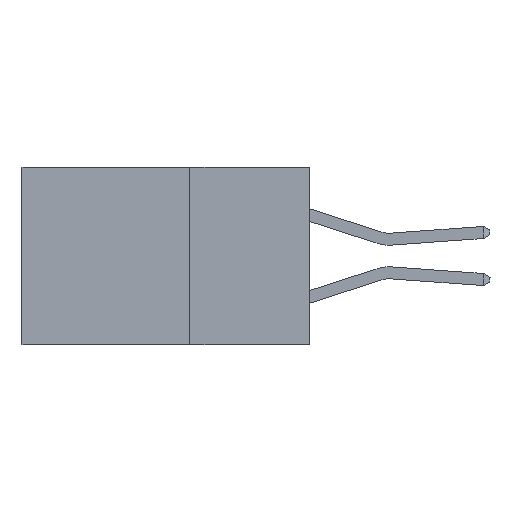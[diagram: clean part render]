
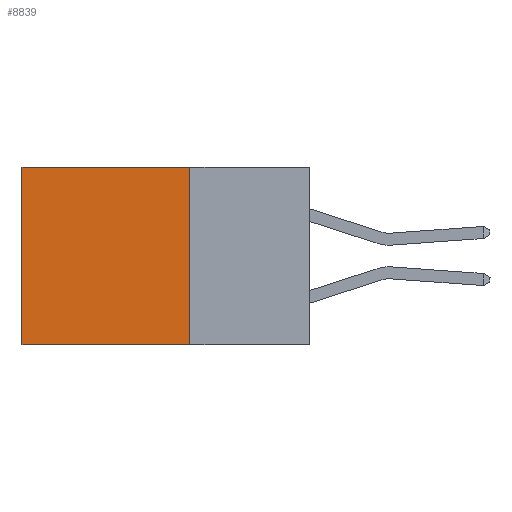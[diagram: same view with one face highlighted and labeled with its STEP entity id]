
A CAD part, left-side view. The second image highlights one B-rep face of the part: STEP entity #8839.
In plain terms, the highlighted planar face has unit normal (-1, 0, 0).
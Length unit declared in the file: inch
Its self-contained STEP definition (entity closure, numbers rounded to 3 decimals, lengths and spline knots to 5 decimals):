
#233 = LINE ( 'NONE', #16346, #13180 ) ;
#2696 = VERTEX_POINT ( 'NONE', #22182 ) ;
#2809 = AXIS2_PLACEMENT_3D ( 'NONE', #17252, #6836, #19024 ) ;
#3231 = EDGE_CURVE ( 'NONE', #2696, #21872, #233, .T. ) ;
#4510 = CARTESIAN_POINT ( 'NONE',  ( 0.2615, 0.25, 0. ) ) ;
#4801 = ORIENTED_EDGE ( 'NONE', *, *, #20707, .T. ) ;
#5436 = LINE ( 'NONE', #20185, #18796 ) ;
#5731 = EDGE_LOOP ( 'NONE', ( #18252, #5789, #15386, #4801 ) ) ;
#5789 = ORIENTED_EDGE ( 'NONE', *, *, #15485, .F. ) ;
#6123 = LINE ( 'NONE', #4510, #10235 ) ;
#6836 = DIRECTION ( 'NONE',  ( 1., 0., 0. ) ) ;
#7475 = CARTESIAN_POINT ( 'NONE',  ( 0.2615, 0.6, -0.37 ) ) ;
#7552 = VECTOR ( 'NONE', #10289, 39.37008 ) ;
#8613 = CARTESIAN_POINT ( 'NONE',  ( 0.2615, 0.25, 0. ) ) ;
#8839 = ADVANCED_FACE ( 'NONE', ( #14628 ), #13788, .F. ) ;
#10235 = VECTOR ( 'NONE', #13327, 39.37008 ) ;
#10289 = DIRECTION ( 'NONE',  ( 0., 0., -1. ) ) ;
#12030 = VERTEX_POINT ( 'NONE', #8613 ) ;
#13180 = VECTOR ( 'NONE', #16242, 39.37008 ) ;
#13327 = DIRECTION ( 'NONE',  ( 0., 1., 0. ) ) ;
#13788 = PLANE ( 'NONE',  #2809 ) ;
#14628 = FACE_OUTER_BOUND ( 'NONE', #5731, .T. ) ;
#15386 = ORIENTED_EDGE ( 'NONE', *, *, #19058, .F. ) ;
#15485 = EDGE_CURVE ( 'NONE', #21978, #21872, #5436, .T. ) ;
#16242 = DIRECTION ( 'NONE',  ( 0., 0., -1. ) ) ;
#16346 = CARTESIAN_POINT ( 'NONE',  ( 0.2615, 0.6, -0.37 ) ) ;
#17252 = CARTESIAN_POINT ( 'NONE',  ( 0.2615, 0.25, -0.37 ) ) ;
#18200 = CARTESIAN_POINT ( 'NONE',  ( 0.2615, 0.25, -0.37 ) ) ;
#18252 = ORIENTED_EDGE ( 'NONE', *, *, #3231, .T. ) ;
#18796 = VECTOR ( 'NONE', #21918, 39.37008 ) ;
#18935 = CARTESIAN_POINT ( 'NONE',  ( 0.2615, 0.25, -0.37 ) ) ;
#19024 = DIRECTION ( 'NONE',  ( 0., 0., -1. ) ) ;
#19058 = EDGE_CURVE ( 'NONE', #12030, #21978, #21972, .T. ) ;
#20185 = CARTESIAN_POINT ( 'NONE',  ( 0.2615, 0.25, -0.37 ) ) ;
#20707 = EDGE_CURVE ( 'NONE', #12030, #2696, #6123, .T. ) ;
#21872 = VERTEX_POINT ( 'NONE', #7475 ) ;
#21918 = DIRECTION ( 'NONE',  ( 0., 1., 0. ) ) ;
#21972 = LINE ( 'NONE', #18935, #7552 ) ;
#21978 = VERTEX_POINT ( 'NONE', #18200 ) ;
#22182 = CARTESIAN_POINT ( 'NONE',  ( 0.2615, 0.6, 0. ) ) ;
